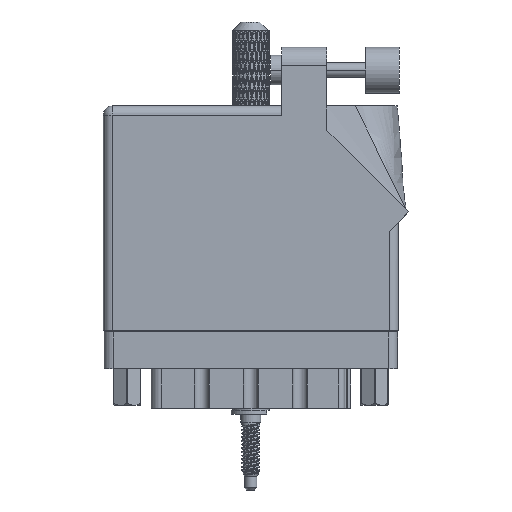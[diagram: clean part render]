
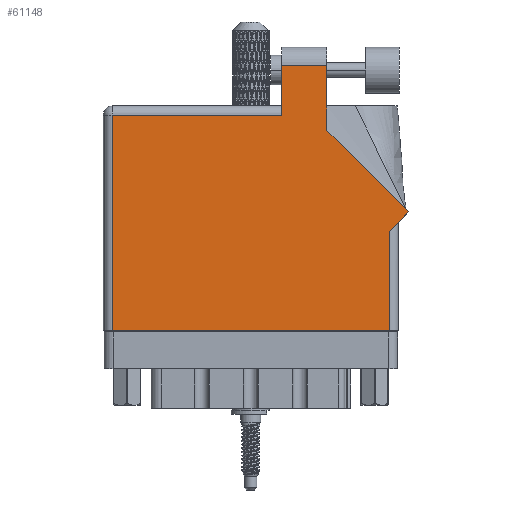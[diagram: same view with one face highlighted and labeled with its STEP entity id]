
A CAD part, front view. The second image highlights one B-rep face of the part: STEP entity #61148.
In plain terms, the highlighted face is planar.
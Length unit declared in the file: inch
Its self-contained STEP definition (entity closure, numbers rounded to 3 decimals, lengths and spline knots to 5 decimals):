
#2693 = EDGE_CURVE ( 'NONE', #63597, #81874, #58542, .T. ) ;
#4010 = EDGE_CURVE ( 'NONE', #81874, #58595, #26032, .T. ) ;
#6399 = CARTESIAN_POINT ( 'NONE',  ( 2.01, 0.737, 0. ) ) ;
#8185 = CARTESIAN_POINT ( 'NONE',  ( 1.524, 1.805, 0. ) ) ;
#8562 = EDGE_CURVE ( 'NONE', #58595, #70112, #26927, .T. ) ;
#8732 = EDGE_CURVE ( 'NONE', #70112, #33148, #20094, .T. ) ;
#11311 = VECTOR ( 'NONE', #101157, 39.37008 ) ;
#11788 = CARTESIAN_POINT ( 'NONE',  ( 0.062, 1.468, 0. ) ) ;
#11950 = CARTESIAN_POINT ( 'NONE',  ( 0.062, 0., 0. ) ) ;
#12366 = EDGE_LOOP ( 'NONE', ( #101318, #71572, #100738, #52009, #45957, #99578, #100511, #77166, #108155 ) ) ;
#16837 = CARTESIAN_POINT ( 'NONE',  ( 1.217, 1.805, 0. ) ) ;
#20094 = LINE ( 'NONE', #102527, #59213 ) ;
#26032 = LINE ( 'NONE', #11950, #78507 ) ;
#26927 = LINE ( 'NONE', #72878, #36327 ) ;
#28952 = DIRECTION ( 'NONE',  ( 0., -1., 0. ) ) ;
#30137 = VERTEX_POINT ( 'NONE', #8185 ) ;
#30425 = VECTOR ( 'NONE', #104297, 39.37008 ) ;
#33148 = VERTEX_POINT ( 'NONE', #88883 ) ;
#36327 = VECTOR ( 'NONE', #37867, 39.37008 ) ;
#37867 = DIRECTION ( 'NONE',  ( 1., 0., 0. ) ) ;
#37931 = DIRECTION ( 'NONE',  ( -0.707, 0.707, 0. ) ) ;
#40563 = VERTEX_POINT ( 'NONE', #91254 ) ;
#42282 = EDGE_CURVE ( 'NONE', #84463, #92126, #63631, .T. ) ;
#45119 = LINE ( 'NONE', #6399, #84015 ) ;
#45957 = ORIENTED_EDGE ( 'NONE', *, *, #4010, .T. ) ;
#46200 = CARTESIAN_POINT ( 'NONE',  ( 1.524, 1.36442, 0. ) ) ;
#46418 = CARTESIAN_POINT ( 'NONE',  ( 0., 1.53, 0. ) ) ;
#47513 = DIRECTION ( 'NONE',  ( 0., 0., -1. ) ) ;
#49151 = DIRECTION ( 'NONE',  ( 0., 1., 0. ) ) ;
#49333 = FACE_OUTER_BOUND ( 'NONE', #12366, .T. ) ;
#52009 = ORIENTED_EDGE ( 'NONE', *, *, #2693, .T. ) ;
#58542 = LINE ( 'NONE', #102264, #11311 ) ;
#58595 = VERTEX_POINT ( 'NONE', #68455 ) ;
#58791 = DIRECTION ( 'NONE',  ( 0., 1., 0. ) ) ;
#59213 = VECTOR ( 'NONE', #58791, 39.37008 ) ;
#61148 = ADVANCED_FACE ( 'NONE', ( #49333 ), #90417, .F. ) ;
#62002 = CARTESIAN_POINT ( 'NONE',  ( 1.948, 0., 0. ) ) ;
#63202 = CARTESIAN_POINT ( 'NONE',  ( 1.217, 1.53, 0. ) ) ;
#63597 = VERTEX_POINT ( 'NONE', #90893 ) ;
#63631 = LINE ( 'NONE', #89509, #79761 ) ;
#66877 = LINE ( 'NONE', #16837, #30425 ) ;
#68455 = CARTESIAN_POINT ( 'NONE',  ( 0.062, 0., 0. ) ) ;
#69772 = VECTOR ( 'NONE', #49151, 39.37008 ) ;
#70112 = VERTEX_POINT ( 'NONE', #62002 ) ;
#70660 = AXIS2_PLACEMENT_3D ( 'NONE', #46418, #47513, #99521 ) ;
#71572 = ORIENTED_EDGE ( 'NONE', *, *, #99981, .T. ) ;
#72878 = CARTESIAN_POINT ( 'NONE',  ( 0., 0., 0. ) ) ;
#74613 = DIRECTION ( 'NONE',  ( 0.707, 0.707, 0. ) ) ;
#75120 = LINE ( 'NONE', #46200, #69772 ) ;
#77166 = ORIENTED_EDGE ( 'NONE', *, *, #100724, .T. ) ;
#77510 = EDGE_CURVE ( 'NONE', #92126, #30137, #75120, .T. ) ;
#78507 = VECTOR ( 'NONE', #89135, 39.37008 ) ;
#79761 = VECTOR ( 'NONE', #37931, 39.37008 ) ;
#81874 = VERTEX_POINT ( 'NONE', #11788 ) ;
#84015 = VECTOR ( 'NONE', #74613, 39.37008 ) ;
#84125 = EDGE_CURVE ( 'NONE', #40563, #63597, #108153, .T. ) ;
#84463 = VERTEX_POINT ( 'NONE', #104829 ) ;
#88883 = CARTESIAN_POINT ( 'NONE',  ( 1.948, 0.675, 0. ) ) ;
#89135 = DIRECTION ( 'NONE',  ( 0., -1., 0. ) ) ;
#89509 = CARTESIAN_POINT ( 'NONE',  ( 2.08071, 0.80771, 0. ) ) ;
#90417 = PLANE ( 'NONE',  #70660 ) ;
#90893 = CARTESIAN_POINT ( 'NONE',  ( 1.217, 1.468, 0. ) ) ;
#91254 = CARTESIAN_POINT ( 'NONE',  ( 1.217, 1.805, 0. ) ) ;
#92126 = VERTEX_POINT ( 'NONE', #103247 ) ;
#93178 = VECTOR ( 'NONE', #28952, 39.37008 ) ;
#99521 = DIRECTION ( 'NONE',  ( -1., 0., 0. ) ) ;
#99578 = ORIENTED_EDGE ( 'NONE', *, *, #8562, .T. ) ;
#99981 = EDGE_CURVE ( 'NONE', #30137, #40563, #66877, .T. ) ;
#100511 = ORIENTED_EDGE ( 'NONE', *, *, #8732, .T. ) ;
#100724 = EDGE_CURVE ( 'NONE', #33148, #84463, #45119, .T. ) ;
#100738 = ORIENTED_EDGE ( 'NONE', *, *, #84125, .T. ) ;
#101157 = DIRECTION ( 'NONE',  ( -1., 0., 0. ) ) ;
#101318 = ORIENTED_EDGE ( 'NONE', *, *, #77510, .T. ) ;
#102264 = CARTESIAN_POINT ( 'NONE',  ( 0., 1.468, 0. ) ) ;
#102527 = CARTESIAN_POINT ( 'NONE',  ( 1.948, 0.737, 0. ) ) ;
#103247 = CARTESIAN_POINT ( 'NONE',  ( 1.524, 1.36442, 0. ) ) ;
#104297 = DIRECTION ( 'NONE',  ( -1., 0., 0. ) ) ;
#104829 = CARTESIAN_POINT ( 'NONE',  ( 2.08071, 0.80771, 0. ) ) ;
#108153 = LINE ( 'NONE', #63202, #93178 ) ;
#108155 = ORIENTED_EDGE ( 'NONE', *, *, #42282, .T. ) ;
